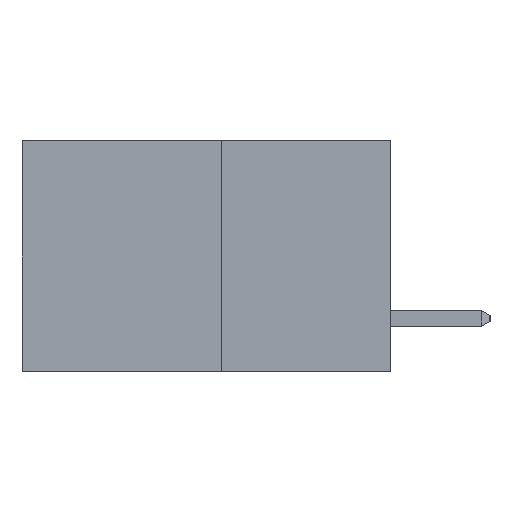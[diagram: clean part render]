
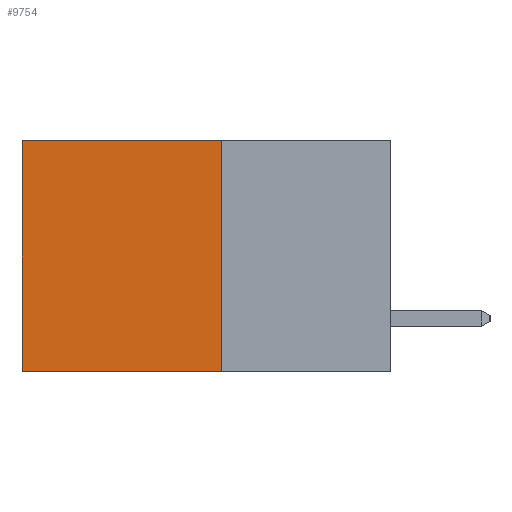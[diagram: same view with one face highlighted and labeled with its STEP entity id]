
A CAD part, left-side view. The second image highlights one B-rep face of the part: STEP entity #9754.
In plain terms, the highlighted planar face has unit normal (-1, 0, 0).
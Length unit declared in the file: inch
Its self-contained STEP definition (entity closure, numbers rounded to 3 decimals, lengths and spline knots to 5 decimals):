
#86 = LINE ( 'NONE', #17552, #18131 ) ;
#515 = ORIENTED_EDGE ( 'NONE', *, *, #18391, .T. ) ;
#990 = CARTESIAN_POINT ( 'NONE',  ( 0.277, 0.59, 0. ) ) ;
#1372 = CARTESIAN_POINT ( 'NONE',  ( 0.277, 0.59, -0.37 ) ) ;
#1541 = DIRECTION ( 'NONE',  ( 1., 0., 0. ) ) ;
#2014 = VERTEX_POINT ( 'NONE', #21197 ) ;
#2732 = LINE ( 'NONE', #11595, #11292 ) ;
#2993 = EDGE_LOOP ( 'NONE', ( #515, #5294, #17922, #9496 ) ) ;
#5121 = VECTOR ( 'NONE', #9821, 39.37008 ) ;
#5294 = ORIENTED_EDGE ( 'NONE', *, *, #7096, .F. ) ;
#6409 = CARTESIAN_POINT ( 'NONE',  ( 0.277, 0.27, -0.37 ) ) ;
#7096 = EDGE_CURVE ( 'NONE', #2014, #18393, #86, .T. ) ;
#7492 = DIRECTION ( 'NONE',  ( 0., 1., 0. ) ) ;
#9496 = ORIENTED_EDGE ( 'NONE', *, *, #13937, .T. ) ;
#9754 = ADVANCED_FACE ( 'NONE', ( #21200 ), #15050, .F. ) ;
#9766 = VERTEX_POINT ( 'NONE', #16755 ) ;
#9821 = DIRECTION ( 'NONE',  ( 0., 0., -1. ) ) ;
#11292 = VECTOR ( 'NONE', #13287, 39.37008 ) ;
#11538 = CARTESIAN_POINT ( 'NONE',  ( 0.277, 0.27, 0. ) ) ;
#11595 = CARTESIAN_POINT ( 'NONE',  ( 0.277, 0.59, -0.37 ) ) ;
#13287 = DIRECTION ( 'NONE',  ( 0., 0., -1. ) ) ;
#13465 = DIRECTION ( 'NONE',  ( 0., 0., -1. ) ) ;
#13937 = EDGE_CURVE ( 'NONE', #9766, #16396, #21743, .T. ) ;
#14544 = EDGE_CURVE ( 'NONE', #9766, #2014, #18558, .T. ) ;
#15050 = PLANE ( 'NONE',  #16409 ) ;
#16396 = VERTEX_POINT ( 'NONE', #990 ) ;
#16409 = AXIS2_PLACEMENT_3D ( 'NONE', #18434, #1541, #13465 ) ;
#16755 = CARTESIAN_POINT ( 'NONE',  ( 0.277, 0.27, 0. ) ) ;
#17552 = CARTESIAN_POINT ( 'NONE',  ( 0.277, 0.27, -0.37 ) ) ;
#17922 = ORIENTED_EDGE ( 'NONE', *, *, #14544, .F. ) ;
#18131 = VECTOR ( 'NONE', #7492, 39.37008 ) ;
#18391 = EDGE_CURVE ( 'NONE', #16396, #18393, #2732, .T. ) ;
#18393 = VERTEX_POINT ( 'NONE', #1372 ) ;
#18434 = CARTESIAN_POINT ( 'NONE',  ( 0.277, 0.27, -0.37 ) ) ;
#18558 = LINE ( 'NONE', #6409, #5121 ) ;
#18850 = VECTOR ( 'NONE', #21573, 39.37008 ) ;
#21197 = CARTESIAN_POINT ( 'NONE',  ( 0.277, 0.27, -0.37 ) ) ;
#21200 = FACE_OUTER_BOUND ( 'NONE', #2993, .T. ) ;
#21573 = DIRECTION ( 'NONE',  ( 0., 1., 0. ) ) ;
#21743 = LINE ( 'NONE', #11538, #18850 ) ;
